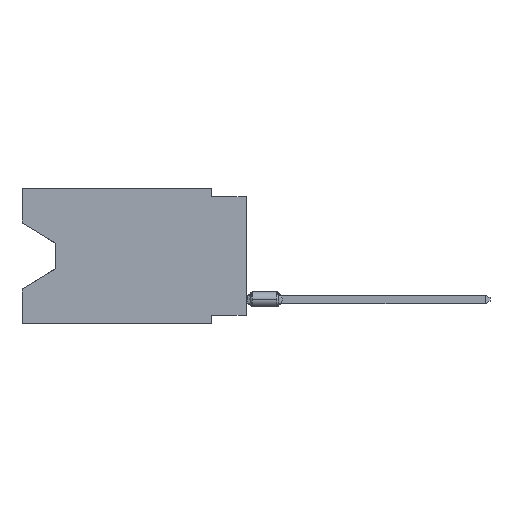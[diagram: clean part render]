
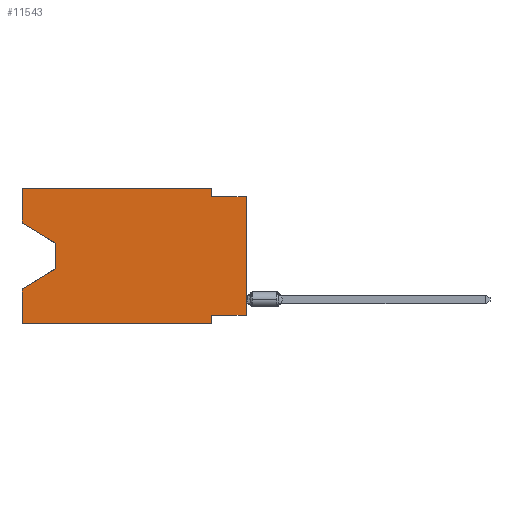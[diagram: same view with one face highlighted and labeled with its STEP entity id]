
A CAD part, left-side view. The second image highlights one B-rep face of the part: STEP entity #11543.
In plain terms, the highlighted planar face has unit normal (-1, 0, 0).
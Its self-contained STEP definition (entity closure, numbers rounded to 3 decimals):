
#62 = DIRECTION ( 'NONE',  ( 0., 0., 1. ) ) ;
#271 = CARTESIAN_POINT ( 'NONE',  ( 0., 0., -9.271 ) ) ;
#762 = LINE ( 'NONE', #17758, #22210 ) ;
#831 = ORIENTED_EDGE ( 'NONE', *, *, #2783, .F. ) ;
#984 = CARTESIAN_POINT ( 'NONE',  ( 0., 16.383, -2.546 ) ) ;
#1100 = VERTEX_POINT ( 'NONE', #2044 ) ;
#2044 = CARTESIAN_POINT ( 'NONE',  ( 0., 2.54, -9.906 ) ) ;
#2077 = ORIENTED_EDGE ( 'NONE', *, *, #7619, .T. ) ;
#2319 = VECTOR ( 'NONE', #12431, 1000. ) ;
#2611 = LINE ( 'NONE', #7596, #22097 ) ;
#2783 = EDGE_CURVE ( 'NONE', #16640, #1100, #17425, .T. ) ;
#3343 = CARTESIAN_POINT ( 'NONE',  ( 0., 16.383, -9.906 ) ) ;
#3403 = DIRECTION ( 'NONE',  ( 0., 0., 1. ) ) ;
#3975 = CARTESIAN_POINT ( 'NONE',  ( 0., 0., -0.635 ) ) ;
#4105 = VERTEX_POINT ( 'NONE', #10828 ) ;
#4371 = CARTESIAN_POINT ( 'NONE',  ( 0., 16.383, -2.546 ) ) ;
#4488 = CARTESIAN_POINT ( 'NONE',  ( 0., 13.97, -5.893 ) ) ;
#4649 = CARTESIAN_POINT ( 'NONE',  ( 0., 13.97, -4.013 ) ) ;
#5017 = CARTESIAN_POINT ( 'NONE',  ( 0., 0., 0. ) ) ;
#5417 = LINE ( 'NONE', #21209, #6256 ) ;
#5497 = VERTEX_POINT ( 'NONE', #21396 ) ;
#5503 = CARTESIAN_POINT ( 'NONE',  ( 0., 2.54, -0.635 ) ) ;
#5725 = EDGE_CURVE ( 'NONE', #14187, #16640, #10572, .T. ) ;
#6011 = CARTESIAN_POINT ( 'NONE',  ( 0., 16.383, 0. ) ) ;
#6127 = DIRECTION ( 'NONE',  ( 0., -1., 0. ) ) ;
#6228 = DIRECTION ( 'NONE',  ( 1., 0., 0. ) ) ;
#6256 = VECTOR ( 'NONE', #9059, 1000. ) ;
#6605 = VERTEX_POINT ( 'NONE', #4649 ) ;
#6621 = CARTESIAN_POINT ( 'NONE',  ( 0., 2.54, -9.271 ) ) ;
#6752 = CARTESIAN_POINT ( 'NONE',  ( 0., 13.97, -5.893 ) ) ;
#6774 = ORIENTED_EDGE ( 'NONE', *, *, #18704, .F. ) ;
#6909 = CARTESIAN_POINT ( 'NONE',  ( 0., 0., -9.271 ) ) ;
#6932 = VECTOR ( 'NONE', #16112, 1000. ) ;
#7144 = DIRECTION ( 'NONE',  ( 0., 1., 0. ) ) ;
#7375 = VERTEX_POINT ( 'NONE', #4488 ) ;
#7445 = VECTOR ( 'NONE', #62, 1000. ) ;
#7596 = CARTESIAN_POINT ( 'NONE',  ( 0., 13.97, -4.013 ) ) ;
#7619 = EDGE_CURVE ( 'NONE', #21292, #1100, #762, .T. ) ;
#7818 = FACE_OUTER_BOUND ( 'NONE', #10900, .T. ) ;
#7828 = LINE ( 'NONE', #21689, #15196 ) ;
#7877 = LINE ( 'NONE', #9816, #17376 ) ;
#8046 = VECTOR ( 'NONE', #18124, 1000. ) ;
#8073 = EDGE_CURVE ( 'NONE', #7375, #4105, #10288, .T. ) ;
#8275 = ORIENTED_EDGE ( 'NONE', *, *, #19019, .T. ) ;
#8341 = AXIS2_PLACEMENT_3D ( 'NONE', #6011, #6228, #12952 ) ;
#8350 = CARTESIAN_POINT ( 'NONE',  ( 0., 2.54, -9.906 ) ) ;
#8854 = CARTESIAN_POINT ( 'NONE',  ( 0., 16.383, 0. ) ) ;
#9059 = DIRECTION ( 'NONE',  ( 0., 0., 1. ) ) ;
#9138 = DIRECTION ( 'NONE',  ( 0., -1., 0. ) ) ;
#9709 = DIRECTION ( 'NONE',  ( 0., 0., -1. ) ) ;
#9816 = CARTESIAN_POINT ( 'NONE',  ( 0., 2.54, 0. ) ) ;
#9882 = VERTEX_POINT ( 'NONE', #984 ) ;
#10288 = LINE ( 'NONE', #6752, #2319 ) ;
#10343 = LINE ( 'NONE', #8854, #16176 ) ;
#10572 = LINE ( 'NONE', #271, #13644 ) ;
#10828 = CARTESIAN_POINT ( 'NONE',  ( 0., 16.383, -7.36 ) ) ;
#10900 = EDGE_LOOP ( 'NONE', ( #17456, #8275, #13962, #21196, #2077, #831, #20672, #17761, #15901, #6774, #16104, #18677 ) ) ;
#11282 = VECTOR ( 'NONE', #20611, 1000. ) ;
#11445 = LINE ( 'NONE', #4371, #8046 ) ;
#11543 = ADVANCED_FACE ( 'NONE', ( #7818 ), #14755, .F. ) ;
#12102 = EDGE_CURVE ( 'NONE', #21292, #4105, #10343, .T. ) ;
#12377 = VERTEX_POINT ( 'NONE', #15303 ) ;
#12431 = DIRECTION ( 'NONE',  ( 0., 0.855, -0.519 ) ) ;
#12952 = DIRECTION ( 'NONE',  ( 0., 0., -1. ) ) ;
#13644 = VECTOR ( 'NONE', #7144, 1000. ) ;
#13962 = ORIENTED_EDGE ( 'NONE', *, *, #8073, .T. ) ;
#14187 = VERTEX_POINT ( 'NONE', #6909 ) ;
#14755 = PLANE ( 'NONE',  #8341 ) ;
#15019 = EDGE_CURVE ( 'NONE', #14187, #20662, #18454, .T. ) ;
#15196 = VECTOR ( 'NONE', #6127, 1000. ) ;
#15303 = CARTESIAN_POINT ( 'NONE',  ( 0., 16.383, 0. ) ) ;
#15901 = ORIENTED_EDGE ( 'NONE', *, *, #21625, .F. ) ;
#15993 = LINE ( 'NONE', #19406, #6932 ) ;
#16104 = ORIENTED_EDGE ( 'NONE', *, *, #20826, .F. ) ;
#16112 = DIRECTION ( 'NONE',  ( 0., -1., 0. ) ) ;
#16176 = VECTOR ( 'NONE', #3403, 1000. ) ;
#16640 = VERTEX_POINT ( 'NONE', #6621 ) ;
#17232 = EDGE_CURVE ( 'NONE', #9882, #6605, #11445, .T. ) ;
#17376 = VECTOR ( 'NONE', #9709, 1000. ) ;
#17425 = LINE ( 'NONE', #8350, #11282 ) ;
#17456 = ORIENTED_EDGE ( 'NONE', *, *, #17232, .T. ) ;
#17758 = CARTESIAN_POINT ( 'NONE',  ( 0., 16.383, -9.906 ) ) ;
#17761 = ORIENTED_EDGE ( 'NONE', *, *, #15019, .T. ) ;
#18124 = DIRECTION ( 'NONE',  ( 0., -0.855, -0.519 ) ) ;
#18155 = DIRECTION ( 'NONE',  ( 0., 0., -1. ) ) ;
#18184 = EDGE_CURVE ( 'NONE', #9882, #12377, #5417, .T. ) ;
#18454 = LINE ( 'NONE', #5017, #7445 ) ;
#18566 = VERTEX_POINT ( 'NONE', #5503 ) ;
#18677 = ORIENTED_EDGE ( 'NONE', *, *, #18184, .F. ) ;
#18704 = EDGE_CURVE ( 'NONE', #5497, #18566, #7877, .T. ) ;
#19019 = EDGE_CURVE ( 'NONE', #6605, #7375, #2611, .T. ) ;
#19406 = CARTESIAN_POINT ( 'NONE',  ( 0., 0., -0.635 ) ) ;
#20611 = DIRECTION ( 'NONE',  ( 0., 0., -1. ) ) ;
#20662 = VERTEX_POINT ( 'NONE', #3975 ) ;
#20672 = ORIENTED_EDGE ( 'NONE', *, *, #5725, .F. ) ;
#20826 = EDGE_CURVE ( 'NONE', #12377, #5497, #7828, .T. ) ;
#21196 = ORIENTED_EDGE ( 'NONE', *, *, #12102, .F. ) ;
#21209 = CARTESIAN_POINT ( 'NONE',  ( 0., 16.383, 0. ) ) ;
#21292 = VERTEX_POINT ( 'NONE', #3343 ) ;
#21396 = CARTESIAN_POINT ( 'NONE',  ( 0., 2.54, 0. ) ) ;
#21625 = EDGE_CURVE ( 'NONE', #18566, #20662, #15993, .T. ) ;
#21689 = CARTESIAN_POINT ( 'NONE',  ( 0., 16.383, 0. ) ) ;
#22097 = VECTOR ( 'NONE', #18155, 1000. ) ;
#22210 = VECTOR ( 'NONE', #9138, 1000. ) ;
